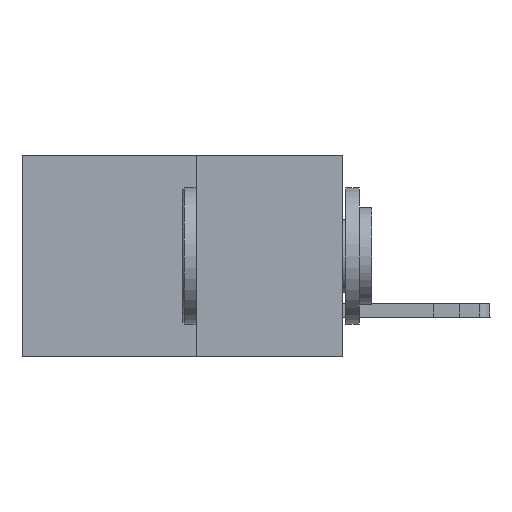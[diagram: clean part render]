
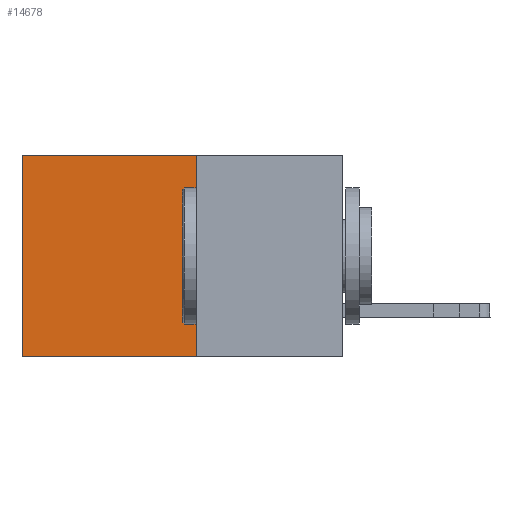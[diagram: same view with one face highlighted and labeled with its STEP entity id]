
A CAD part, left-side view. The second image highlights one B-rep face of the part: STEP entity #14678.
In plain terms, the highlighted planar face has unit normal (-1, 0, 0).
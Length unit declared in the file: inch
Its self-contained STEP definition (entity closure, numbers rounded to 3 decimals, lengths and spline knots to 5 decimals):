
#1866 = CARTESIAN_POINT ( 'NONE',  ( 0.277, 0.59, -0.37 ) ) ;
#2244 = DIRECTION ( 'NONE',  ( 0., 0., -1. ) ) ;
#2622 = CARTESIAN_POINT ( 'NONE',  ( 0.277, 0.27, 0. ) ) ;
#3577 = VECTOR ( 'NONE', #25344, 39.37008 ) ;
#3579 = CARTESIAN_POINT ( 'NONE',  ( 0.277, 0.27, 0. ) ) ;
#3823 = DIRECTION ( 'NONE',  ( 0., 0., -1. ) ) ;
#4980 = DIRECTION ( 'NONE',  ( 1., 0., 0. ) ) ;
#5259 = VECTOR ( 'NONE', #2244, 39.37008 ) ;
#7140 = PLANE ( 'NONE',  #10840 ) ;
#7928 = ORIENTED_EDGE ( 'NONE', *, *, #11504, .F. ) ;
#8472 = VECTOR ( 'NONE', #19030, 39.37008 ) ;
#10027 = CARTESIAN_POINT ( 'NONE',  ( 0.277, 0.27, -0.37 ) ) ;
#10036 = VERTEX_POINT ( 'NONE', #10767 ) ;
#10380 = ORIENTED_EDGE ( 'NONE', *, *, #11278, .T. ) ;
#10767 = CARTESIAN_POINT ( 'NONE',  ( 0.277, 0.59, 0. ) ) ;
#10840 = AXIS2_PLACEMENT_3D ( 'NONE', #15957, #4980, #20437 ) ;
#11278 = EDGE_CURVE ( 'NONE', #21073, #10036, #23366, .T. ) ;
#11504 = EDGE_CURVE ( 'NONE', #21073, #24006, #24933, .T. ) ;
#12759 = ORIENTED_EDGE ( 'NONE', *, *, #17319, .F. ) ;
#14678 = ADVANCED_FACE ( 'NONE', ( #18122 ), #7140, .F. ) ;
#15957 = CARTESIAN_POINT ( 'NONE',  ( 0.277, 0.27, -0.37 ) ) ;
#16957 = CARTESIAN_POINT ( 'NONE',  ( 0.277, 0.59, -0.37 ) ) ;
#17319 = EDGE_CURVE ( 'NONE', #24006, #25822, #20430, .T. ) ;
#17698 = CARTESIAN_POINT ( 'NONE',  ( 0.277, 0.27, -0.37 ) ) ;
#18122 = FACE_OUTER_BOUND ( 'NONE', #21034, .T. ) ;
#19030 = DIRECTION ( 'NONE',  ( 0., 1., 0. ) ) ;
#19075 = ORIENTED_EDGE ( 'NONE', *, *, #19865, .T. ) ;
#19132 = LINE ( 'NONE', #16957, #23586 ) ;
#19865 = EDGE_CURVE ( 'NONE', #10036, #25822, #19132, .T. ) ;
#19890 = CARTESIAN_POINT ( 'NONE',  ( 0.277, 0.27, -0.37 ) ) ;
#20430 = LINE ( 'NONE', #10027, #3577 ) ;
#20437 = DIRECTION ( 'NONE',  ( 0., 0., -1. ) ) ;
#21034 = EDGE_LOOP ( 'NONE', ( #19075, #12759, #7928, #10380 ) ) ;
#21073 = VERTEX_POINT ( 'NONE', #2622 ) ;
#23366 = LINE ( 'NONE', #3579, #8472 ) ;
#23586 = VECTOR ( 'NONE', #3823, 39.37008 ) ;
#24006 = VERTEX_POINT ( 'NONE', #19890 ) ;
#24933 = LINE ( 'NONE', #17698, #5259 ) ;
#25344 = DIRECTION ( 'NONE',  ( 0., 1., 0. ) ) ;
#25822 = VERTEX_POINT ( 'NONE', #1866 ) ;
